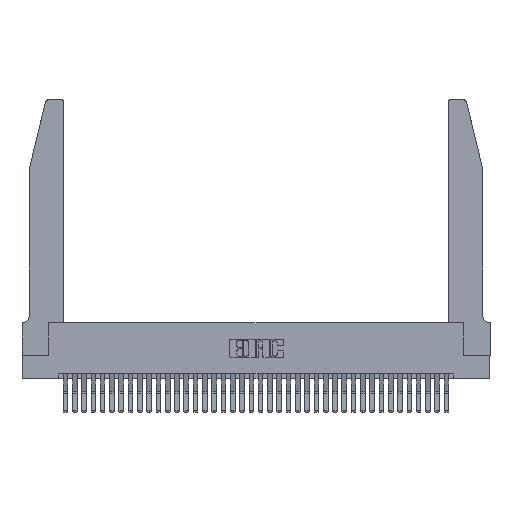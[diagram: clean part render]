
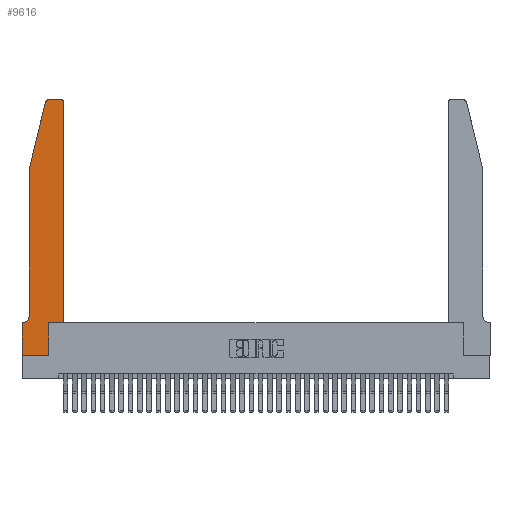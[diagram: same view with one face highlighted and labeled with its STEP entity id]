
A CAD part, top view. The second image highlights one B-rep face of the part: STEP entity #9616.
In plain terms, the highlighted planar face has unit normal (0, 0, 1).
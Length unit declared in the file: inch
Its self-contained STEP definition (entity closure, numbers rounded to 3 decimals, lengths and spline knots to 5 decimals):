
#672 = DIRECTION ( 'NONE',  ( -1., 0., 0. ) ) ;
#836 = VERTEX_POINT ( 'NONE', #24792 ) ;
#1234 = EDGE_CURVE ( 'NONE', #10401, #34603, #17384, .T. ) ;
#1364 = EDGE_CURVE ( 'NONE', #17053, #28283, #24213, .T. ) ;
#1388 = DIRECTION ( 'NONE',  ( -1., 0., 0. ) ) ;
#1405 = DIRECTION ( 'NONE',  ( 0., -1., 0. ) ) ;
#1609 = CARTESIAN_POINT ( 'NONE',  ( 0.2865, 0., 0.37 ) ) ;
#1944 = CARTESIAN_POINT ( 'NONE',  ( 0.25487, 2.72718, 0.37 ) ) ;
#3816 = LINE ( 'NONE', #25462, #28057 ) ;
#4099 = VECTOR ( 'NONE', #8354, 39.37008 ) ;
#4223 = VERTEX_POINT ( 'NONE', #6884 ) ;
#4338 = ORIENTED_EDGE ( 'NONE', *, *, #9286, .T. ) ;
#4380 = PLANE ( 'NONE',  #31507 ) ;
#4439 = LINE ( 'NONE', #8498, #13587 ) ;
#4477 = VECTOR ( 'NONE', #28294, 39.37008 ) ;
#5634 = DIRECTION ( 'NONE',  ( 1., 0., 0. ) ) ;
#5699 = VERTEX_POINT ( 'NONE', #26147 ) ;
#5820 = DIRECTION ( 'NONE',  ( -1., 0., 0. ) ) ;
#6092 = VERTEX_POINT ( 'NONE', #14149 ) ;
#6504 = VERTEX_POINT ( 'NONE', #20365 ) ;
#6884 = CARTESIAN_POINT ( 'NONE',  ( 0.0055, 0.35, 0.37 ) ) ;
#7200 = ORIENTED_EDGE ( 'NONE', *, *, #24029, .T. ) ;
#7554 = EDGE_CURVE ( 'NONE', #5699, #836, #3816, .T. ) ;
#7724 = CARTESIAN_POINT ( 'NONE',  ( 0.2865, 0.35, 0.37 ) ) ;
#7866 = AXIS2_PLACEMENT_3D ( 'NONE', #35723, #18099, #672 ) ;
#8082 = EDGE_CURVE ( 'NONE', #34603, #10166, #21135, .T. ) ;
#8083 = VERTEX_POINT ( 'NONE', #19358 ) ;
#8354 = DIRECTION ( 'NONE',  ( 1., 0., 0. ) ) ;
#8377 = EDGE_CURVE ( 'NONE', #8083, #6092, #18848, .T. ) ;
#8498 = CARTESIAN_POINT ( 'NONE',  ( 0.0755, 0.35, 0.37 ) ) ;
#9286 = EDGE_CURVE ( 'NONE', #6504, #17053, #20145, .T. ) ;
#9411 = EDGE_LOOP ( 'NONE', ( #25780, #7200, #13505, #16917, #14906, #17698, #4338, #11353, #35520, #23751, #19589, #19186 ) ) ;
#9616 = ADVANCED_FACE ( 'NONE', ( #22384 ), #4380, .T. ) ;
#9830 = LINE ( 'NONE', #25664, #37274 ) ;
#10166 = VERTEX_POINT ( 'NONE', #30997 ) ;
#10401 = VERTEX_POINT ( 'NONE', #7724 ) ;
#10926 = VERTEX_POINT ( 'NONE', #1944 ) ;
#11353 = ORIENTED_EDGE ( 'NONE', *, *, #1364, .T. ) ;
#13369 = VECTOR ( 'NONE', #33966, 39.37008 ) ;
#13505 = ORIENTED_EDGE ( 'NONE', *, *, #19223, .T. ) ;
#13522 = CARTESIAN_POINT ( 'NONE',  ( 0., 0., 0.37 ) ) ;
#13587 = VECTOR ( 'NONE', #5820, 39.37008 ) ;
#13818 = VECTOR ( 'NONE', #1388, 39.37008 ) ;
#14149 = CARTESIAN_POINT ( 'NONE',  ( 0.284, 2.75, 0.37 ) ) ;
#14906 = ORIENTED_EDGE ( 'NONE', *, *, #27584, .T. ) ;
#16612 = DIRECTION ( 'NONE',  ( 1., 0., 0. ) ) ;
#16917 = ORIENTED_EDGE ( 'NONE', *, *, #7554, .T. ) ;
#17053 = VERTEX_POINT ( 'NONE', #13522 ) ;
#17384 = LINE ( 'NONE', #25941, #20127 ) ;
#17698 = ORIENTED_EDGE ( 'NONE', *, *, #34326, .T. ) ;
#18099 = DIRECTION ( 'NONE',  ( 0., 0., -1. ) ) ;
#18161 = EDGE_CURVE ( 'NONE', #28283, #10401, #20009, .T. ) ;
#18447 = AXIS2_PLACEMENT_3D ( 'NONE', #27452, #36647, #30226 ) ;
#18848 = LINE ( 'NONE', #18896, #13818 ) ;
#18896 = CARTESIAN_POINT ( 'NONE',  ( 0.2605, 2.75, 0.37 ) ) ;
#19179 = DIRECTION ( 'NONE',  ( 0., 0., 1. ) ) ;
#19186 = ORIENTED_EDGE ( 'NONE', *, *, #30253, .T. ) ;
#19223 = EDGE_CURVE ( 'NONE', #10926, #5699, #9830, .T. ) ;
#19230 = CARTESIAN_POINT ( 'NONE',  ( 0.4505, 0.35, 0.37 ) ) ;
#19358 = CARTESIAN_POINT ( 'NONE',  ( 0.4205, 2.75, 0.37 ) ) ;
#19589 = ORIENTED_EDGE ( 'NONE', *, *, #8082, .T. ) ;
#19820 = CARTESIAN_POINT ( 'NONE',  ( 0.284, 2.72, 0.37 ) ) ;
#19958 = CARTESIAN_POINT ( 'NONE',  ( 0., 0., 0.37 ) ) ;
#20009 = LINE ( 'NONE', #28172, #4477 ) ;
#20127 = VECTOR ( 'NONE', #5634, 39.37008 ) ;
#20145 = LINE ( 'NONE', #22221, #37503 ) ;
#20365 = CARTESIAN_POINT ( 'NONE',  ( 0., 0.35, 0.37 ) ) ;
#21021 = AXIS2_PLACEMENT_3D ( 'NONE', #19820, #25210, #16612 ) ;
#21135 = LINE ( 'NONE', #19230, #13369 ) ;
#22221 = CARTESIAN_POINT ( 'NONE',  ( 0., 0., 0.37 ) ) ;
#22384 = FACE_OUTER_BOUND ( 'NONE', #9411, .T. ) ;
#23225 = CIRCLE ( 'NONE', #18447, 0.03 ) ;
#23751 = ORIENTED_EDGE ( 'NONE', *, *, #1234, .T. ) ;
#24029 = EDGE_CURVE ( 'NONE', #6092, #10926, #28836, .T. ) ;
#24213 = LINE ( 'NONE', #19958, #4099 ) ;
#24792 = CARTESIAN_POINT ( 'NONE',  ( 0.0755, 0.42, 0.37 ) ) ;
#24798 = CARTESIAN_POINT ( 'NONE',  ( 0., 0.35, 0.37 ) ) ;
#25210 = DIRECTION ( 'NONE',  ( 0., 0., 1. ) ) ;
#25462 = CARTESIAN_POINT ( 'NONE',  ( 0.0755, 2., 0.37 ) ) ;
#25664 = CARTESIAN_POINT ( 'NONE',  ( 0.0755, 2., 0.37 ) ) ;
#25780 = ORIENTED_EDGE ( 'NONE', *, *, #8377, .T. ) ;
#25941 = CARTESIAN_POINT ( 'NONE',  ( 0.4505, 0.35, 0.37 ) ) ;
#26147 = CARTESIAN_POINT ( 'NONE',  ( 0.0755, 2., 0.37 ) ) ;
#27452 = CARTESIAN_POINT ( 'NONE',  ( 0.4205, 2.72, 0.37 ) ) ;
#27584 = EDGE_CURVE ( 'NONE', #836, #4223, #34386, .T. ) ;
#28057 = VECTOR ( 'NONE', #31333, 39.37008 ) ;
#28172 = CARTESIAN_POINT ( 'NONE',  ( 0.2865, 0.35, 0.37 ) ) ;
#28283 = VERTEX_POINT ( 'NONE', #1609 ) ;
#28294 = DIRECTION ( 'NONE',  ( 0., 1., 0. ) ) ;
#28836 = CIRCLE ( 'NONE', #21021, 0.03 ) ;
#30226 = DIRECTION ( 'NONE',  ( 1., 0., 0. ) ) ;
#30253 = EDGE_CURVE ( 'NONE', #10166, #8083, #23225, .T. ) ;
#30997 = CARTESIAN_POINT ( 'NONE',  ( 0.4505, 2.72, 0.37 ) ) ;
#31333 = DIRECTION ( 'NONE',  ( 0., -1., 0. ) ) ;
#31507 = AXIS2_PLACEMENT_3D ( 'NONE', #24798, #19179, #33645 ) ;
#33645 = DIRECTION ( 'NONE',  ( 1., 0., 0. ) ) ;
#33966 = DIRECTION ( 'NONE',  ( 0., 1., 0. ) ) ;
#34326 = EDGE_CURVE ( 'NONE', #4223, #6504, #4439, .T. ) ;
#34386 = CIRCLE ( 'NONE', #7866, 0.07 ) ;
#34603 = VERTEX_POINT ( 'NONE', #36293 ) ;
#35283 = DIRECTION ( 'NONE',  ( -0.239, -0.971, 0. ) ) ;
#35520 = ORIENTED_EDGE ( 'NONE', *, *, #18161, .T. ) ;
#35723 = CARTESIAN_POINT ( 'NONE',  ( 0.0055, 0.42, 0.37 ) ) ;
#36293 = CARTESIAN_POINT ( 'NONE',  ( 0.4505, 0.35, 0.37 ) ) ;
#36647 = DIRECTION ( 'NONE',  ( 0., 0., 1. ) ) ;
#37274 = VECTOR ( 'NONE', #35283, 39.37008 ) ;
#37503 = VECTOR ( 'NONE', #1405, 39.37008 ) ;
